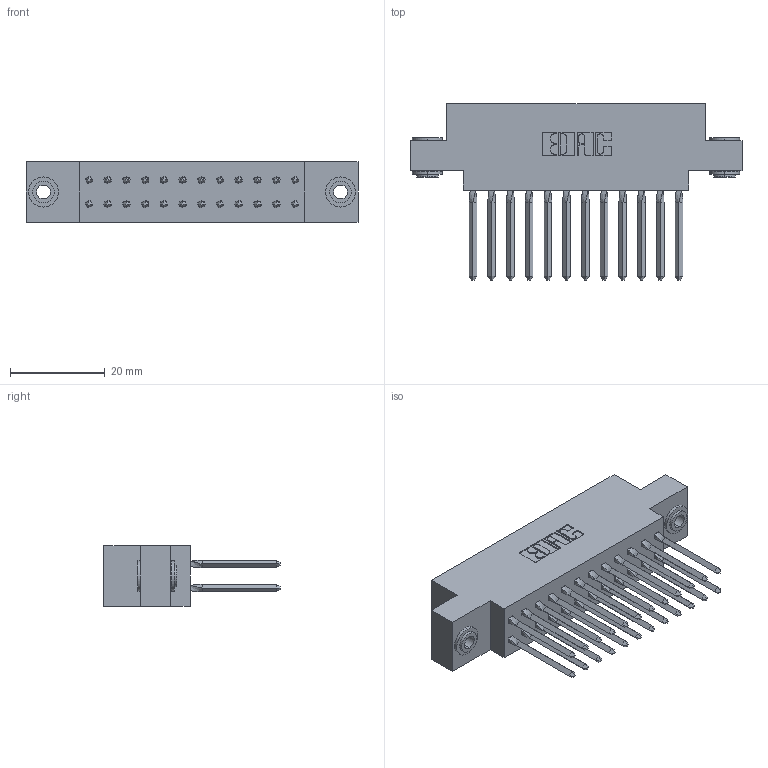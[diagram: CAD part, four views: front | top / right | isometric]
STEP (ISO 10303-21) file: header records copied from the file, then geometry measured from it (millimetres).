
FILE_DESCRIPTION (( 'STEP AP203' ), '1' );
FILE_NAME ('317-024-542-803.STEP', '2020-02-27T18:11:12', ( '' ), ( '' ), 'SwSTEP 2.0', 'SolidWorks 2016', '' );
FILE_SCHEMA (( 'CONFIG_CONTROL_DESIGN' ));
Length unit declared in the file: inch
Products named in the file (4): 317 Part_.156 Dia - TH; 345-250-002_345-250-002-102; 317-290-003_542; 317-024-542-803
Assembly tree (27 placements, depth 2):
  317-024-542-803
    317 Part_.156 Dia - TH
    317-290-003_542  x24
    345-250-002_345-250-002-102  x2
Bounding box: 70.26 x 37.34 x 12.7 mm (x, y, z)
Volume: 10575.6 mm3; surface area: 13959.9 mm2
Topology: 27 solids, 27 shells, 1508 faces, 4191 edges, 2678 vertices
Faces by surface type: plane 1172, cylinder 232, bspline 96, cone 8
Entity records: 21198 total; most frequent: CARTESIAN_POINT 3912, ORIENTED_EDGE 3568, DIRECTION 3094, EDGE_CURVE 1784, VECTOR 1590, LINE 1590, VERTEX_POINT 1182, AXIS2_PLACEMENT_3D 752
